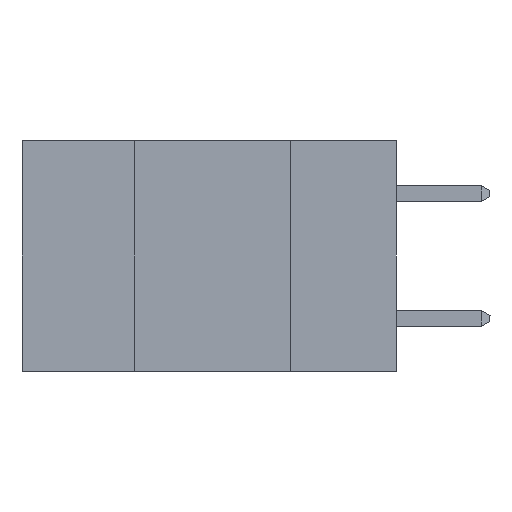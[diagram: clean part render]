
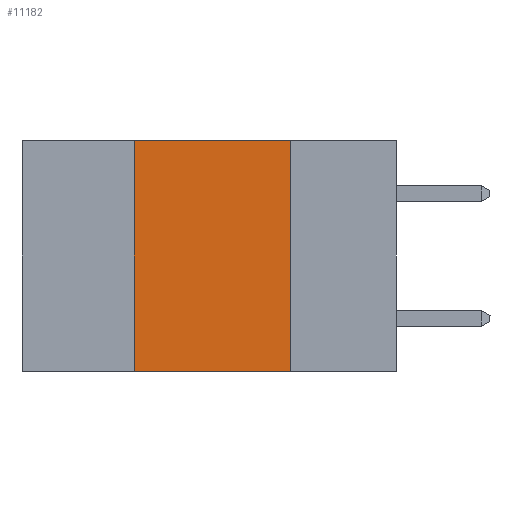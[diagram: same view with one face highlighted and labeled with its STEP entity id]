
A CAD part, left-side view. The second image highlights one B-rep face of the part: STEP entity #11182.
In plain terms, the highlighted planar face has unit normal (-1, 0, 0).
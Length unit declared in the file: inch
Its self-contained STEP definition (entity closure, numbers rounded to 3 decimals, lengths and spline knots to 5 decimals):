
#39 = LINE ( 'NONE', #16963, #17295 ) ;
#59 = LINE ( 'NONE', #1932, #8856 ) ;
#1932 = CARTESIAN_POINT ( 'NONE',  ( 0., 0.42, -0.37 ) ) ;
#2978 = DIRECTION ( 'NONE',  ( 0., 0., -1. ) ) ;
#3212 = PLANE ( 'NONE',  #21678 ) ;
#3466 = CARTESIAN_POINT ( 'NONE',  ( 0., 0.6, -0.37 ) ) ;
#3703 = DIRECTION ( 'NONE',  ( 0., 0., 1. ) ) ;
#4051 = FACE_OUTER_BOUND ( 'NONE', #6951, .T. ) ;
#4230 = CARTESIAN_POINT ( 'NONE',  ( 0., 0.17, -0.37 ) ) ;
#6668 = LINE ( 'NONE', #3466, #15730 ) ;
#6827 = EDGE_CURVE ( 'NONE', #21929, #7096, #6668, .T. ) ;
#6866 = LINE ( 'NONE', #11606, #10868 ) ;
#6951 = EDGE_LOOP ( 'NONE', ( #7428, #11972, #14113, #19579 ) ) ;
#7096 = VERTEX_POINT ( 'NONE', #4230 ) ;
#7428 = ORIENTED_EDGE ( 'NONE', *, *, #9142, .F. ) ;
#8502 = CARTESIAN_POINT ( 'NONE',  ( 0., 0.6, 0. ) ) ;
#8532 = DIRECTION ( 'NONE',  ( 0., -1., 0. ) ) ;
#8856 = VECTOR ( 'NONE', #3703, 39.37008 ) ;
#8875 = VERTEX_POINT ( 'NONE', #16074 ) ;
#9142 = EDGE_CURVE ( 'NONE', #8875, #7096, #6866, .T. ) ;
#10868 = VECTOR ( 'NONE', #2978, 39.37008 ) ;
#11182 = ADVANCED_FACE ( 'NONE', ( #4051 ), #3212, .F. ) ;
#11606 = CARTESIAN_POINT ( 'NONE',  ( 0., 0.17, -0.37 ) ) ;
#11922 = DIRECTION ( 'NONE',  ( 0., 0., -1. ) ) ;
#11972 = ORIENTED_EDGE ( 'NONE', *, *, #14828, .F. ) ;
#12785 = CARTESIAN_POINT ( 'NONE',  ( 0., 0.42, -0.37 ) ) ;
#14113 = ORIENTED_EDGE ( 'NONE', *, *, #19716, .F. ) ;
#14828 = EDGE_CURVE ( 'NONE', #18144, #8875, #39, .T. ) ;
#15730 = VECTOR ( 'NONE', #17254, 39.37008 ) ;
#16074 = CARTESIAN_POINT ( 'NONE',  ( 0., 0.17, 0. ) ) ;
#16963 = CARTESIAN_POINT ( 'NONE',  ( 0., 0.6, 0. ) ) ;
#17254 = DIRECTION ( 'NONE',  ( 0., -1., 0. ) ) ;
#17295 = VECTOR ( 'NONE', #8532, 39.37008 ) ;
#18144 = VERTEX_POINT ( 'NONE', #21734 ) ;
#19579 = ORIENTED_EDGE ( 'NONE', *, *, #6827, .T. ) ;
#19716 = EDGE_CURVE ( 'NONE', #21929, #18144, #59, .T. ) ;
#21678 = AXIS2_PLACEMENT_3D ( 'NONE', #8502, #21893, #11922 ) ;
#21734 = CARTESIAN_POINT ( 'NONE',  ( 0., 0.42, 0. ) ) ;
#21893 = DIRECTION ( 'NONE',  ( 1., 0., 0. ) ) ;
#21929 = VERTEX_POINT ( 'NONE', #12785 ) ;
